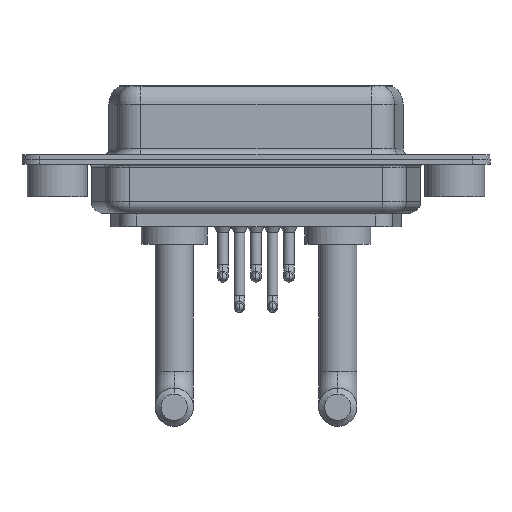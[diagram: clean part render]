
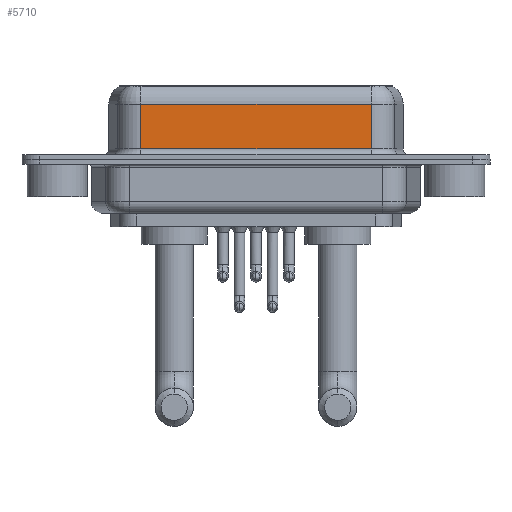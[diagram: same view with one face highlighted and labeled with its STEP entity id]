
A CAD part, front view. The second image highlights one B-rep face of the part: STEP entity #5710.
In plain terms, the highlighted planar face has unit normal (0, -1, 0).
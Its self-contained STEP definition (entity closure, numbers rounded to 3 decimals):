
#799 = DIRECTION ( 'NONE',  ( 0., 0., -1. ) ) ;
#1706 = DIRECTION ( 'NONE',  ( 1., 0., 0. ) ) ;
#1722 = DIRECTION ( 'NONE',  ( -1., 0., 0. ) ) ;
#1740 = AXIS2_PLACEMENT_3D ( 'NONE', #14192, #11431, #2696 ) ;
#1980 = VECTOR ( 'NONE', #1722, 1000. ) ;
#2696 = DIRECTION ( 'NONE',  ( 0., 0., 1. ) ) ;
#3002 = CARTESIAN_POINT ( 'NONE',  ( 26.287, -3.95, 4.65 ) ) ;
#3597 = LINE ( 'NONE', #4956, #14314 ) ;
#4758 = VERTEX_POINT ( 'NONE', #15347 ) ;
#4848 = ORIENTED_EDGE ( 'NONE', *, *, #12904, .T. ) ;
#4956 = CARTESIAN_POINT ( 'NONE',  ( 26.287, -3.95, 6.4 ) ) ;
#5191 = ORIENTED_EDGE ( 'NONE', *, *, #11008, .T. ) ;
#5710 = ADVANCED_FACE ( 'NONE', ( #11516 ), #10349, .F. ) ;
#5770 = EDGE_CURVE ( 'NONE', #14717, #14578, #11607, .T. ) ;
#5853 = CARTESIAN_POINT ( 'NONE',  ( 7.013, -3.95, 0.9 ) ) ;
#8128 = ORIENTED_EDGE ( 'NONE', *, *, #13914, .F. ) ;
#9005 = CARTESIAN_POINT ( 'NONE',  ( 26.287, -3.95, 4.65 ) ) ;
#9060 = LINE ( 'NONE', #3002, #1980 ) ;
#10349 = PLANE ( 'NONE',  #1740 ) ;
#10899 = CARTESIAN_POINT ( 'NONE',  ( 26.287, -3.95, 0.9 ) ) ;
#11008 = EDGE_CURVE ( 'NONE', #14868, #14717, #9060, .T. ) ;
#11431 = DIRECTION ( 'NONE',  ( 0., 1., 0. ) ) ;
#11516 = FACE_OUTER_BOUND ( 'NONE', #12402, .T. ) ;
#11528 = CARTESIAN_POINT ( 'NONE',  ( 7.013, -3.95, 4.65 ) ) ;
#11607 = LINE ( 'NONE', #16825, #14545 ) ;
#12095 = VECTOR ( 'NONE', #1706, 1000. ) ;
#12402 = EDGE_LOOP ( 'NONE', ( #8128, #5191, #14313, #4848 ) ) ;
#12904 = EDGE_CURVE ( 'NONE', #14578, #4758, #14671, .T. ) ;
#13914 = EDGE_CURVE ( 'NONE', #14868, #4758, #3597, .T. ) ;
#14192 = CARTESIAN_POINT ( 'NONE',  ( 26.287, -3.95, 6.4 ) ) ;
#14313 = ORIENTED_EDGE ( 'NONE', *, *, #5770, .T. ) ;
#14314 = VECTOR ( 'NONE', #799, 1000. ) ;
#14545 = VECTOR ( 'NONE', #15548, 1000. ) ;
#14578 = VERTEX_POINT ( 'NONE', #5853 ) ;
#14671 = LINE ( 'NONE', #10899, #12095 ) ;
#14717 = VERTEX_POINT ( 'NONE', #11528 ) ;
#14868 = VERTEX_POINT ( 'NONE', #9005 ) ;
#15347 = CARTESIAN_POINT ( 'NONE',  ( 26.287, -3.95, 0.9 ) ) ;
#15548 = DIRECTION ( 'NONE',  ( 0., 0., -1. ) ) ;
#16825 = CARTESIAN_POINT ( 'NONE',  ( 7.013, -3.95, 6.4 ) ) ;
